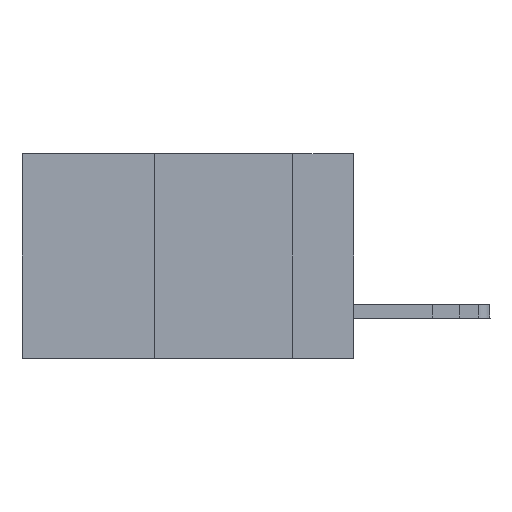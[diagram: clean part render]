
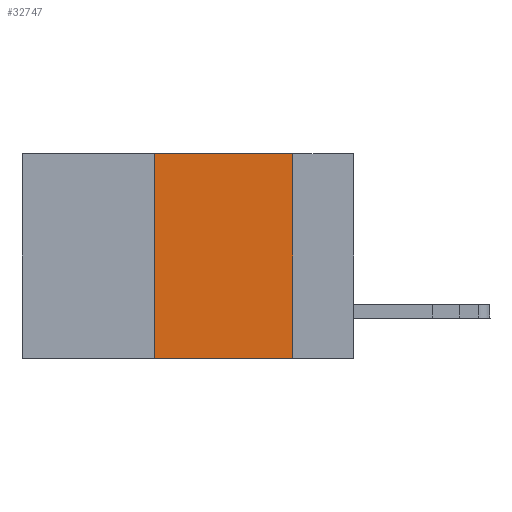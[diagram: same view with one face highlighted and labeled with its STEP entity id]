
A CAD part, left-side view. The second image highlights one B-rep face of the part: STEP entity #32747.
In plain terms, the highlighted planar face has unit normal (-1, 0, 0).
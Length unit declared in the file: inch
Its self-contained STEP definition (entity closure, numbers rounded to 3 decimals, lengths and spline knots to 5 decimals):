
#946 = VERTEX_POINT ( 'NONE', #32536 ) ;
#1290 = ORIENTED_EDGE ( 'NONE', *, *, #9206, .T. ) ;
#2220 = AXIS2_PLACEMENT_3D ( 'NONE', #30879, #22362, #5160 ) ;
#2301 = CARTESIAN_POINT ( 'NONE',  ( 0., 0.36, -0.37 ) ) ;
#3493 = CARTESIAN_POINT ( 'NONE',  ( 0., 0.36, 0. ) ) ;
#4574 = VERTEX_POINT ( 'NONE', #13065 ) ;
#5160 = DIRECTION ( 'NONE',  ( 0., 0., -1. ) ) ;
#6979 = VECTOR ( 'NONE', #20688, 39.37008 ) ;
#8782 = LINE ( 'NONE', #3493, #6979 ) ;
#9182 = CARTESIAN_POINT ( 'NONE',  ( 0., 0.11, -0.37 ) ) ;
#9206 = EDGE_CURVE ( 'NONE', #23872, #33396, #32425, .T. ) ;
#11715 = ORIENTED_EDGE ( 'NONE', *, *, #12347, .F. ) ;
#12347 = EDGE_CURVE ( 'NONE', #23872, #946, #8782, .T. ) ;
#13065 = CARTESIAN_POINT ( 'NONE',  ( 0., 0.11, 0. ) ) ;
#13650 = LINE ( 'NONE', #17342, #27998 ) ;
#13867 = LINE ( 'NONE', #30935, #20582 ) ;
#14081 = DIRECTION ( 'NONE',  ( 0., -1., 0. ) ) ;
#15939 = FACE_OUTER_BOUND ( 'NONE', #33622, .T. ) ;
#16658 = DIRECTION ( 'NONE',  ( 0., 0., -1. ) ) ;
#17342 = CARTESIAN_POINT ( 'NONE',  ( 0., 0.6, 0. ) ) ;
#19457 = PLANE ( 'NONE',  #2220 ) ;
#20582 = VECTOR ( 'NONE', #16658, 39.37008 ) ;
#20688 = DIRECTION ( 'NONE',  ( 0., 0., 1. ) ) ;
#20860 = ORIENTED_EDGE ( 'NONE', *, *, #26919, .F. ) ;
#21143 = EDGE_CURVE ( 'NONE', #4574, #33396, #13867, .T. ) ;
#22362 = DIRECTION ( 'NONE',  ( 1., 0., 0. ) ) ;
#23241 = DIRECTION ( 'NONE',  ( 0., -1., 0. ) ) ;
#23872 = VERTEX_POINT ( 'NONE', #2301 ) ;
#25818 = ORIENTED_EDGE ( 'NONE', *, *, #21143, .F. ) ;
#26919 = EDGE_CURVE ( 'NONE', #946, #4574, #13650, .T. ) ;
#27998 = VECTOR ( 'NONE', #23241, 39.37008 ) ;
#28381 = CARTESIAN_POINT ( 'NONE',  ( 0., 0.6, -0.37 ) ) ;
#30879 = CARTESIAN_POINT ( 'NONE',  ( 0., 0.6, 0. ) ) ;
#30935 = CARTESIAN_POINT ( 'NONE',  ( 0., 0.11, 0. ) ) ;
#31541 = VECTOR ( 'NONE', #14081, 39.37008 ) ;
#32425 = LINE ( 'NONE', #28381, #31541 ) ;
#32536 = CARTESIAN_POINT ( 'NONE',  ( 0., 0.36, 0. ) ) ;
#32747 = ADVANCED_FACE ( 'NONE', ( #15939 ), #19457, .F. ) ;
#33396 = VERTEX_POINT ( 'NONE', #9182 ) ;
#33622 = EDGE_LOOP ( 'NONE', ( #25818, #20860, #11715, #1290 ) ) ;
